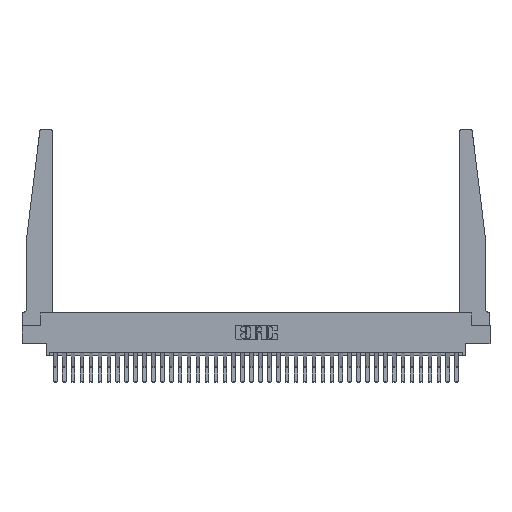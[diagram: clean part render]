
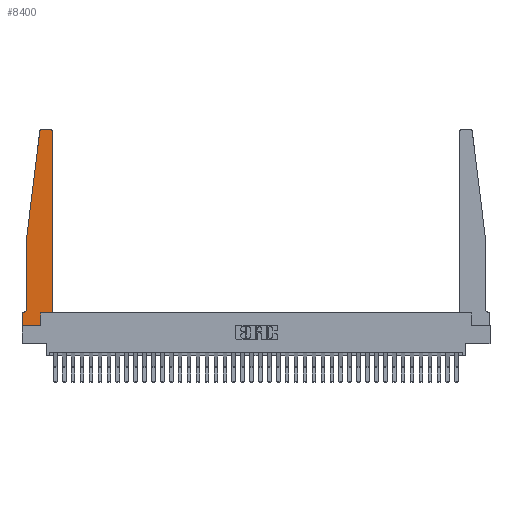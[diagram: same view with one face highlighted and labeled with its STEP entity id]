
A CAD part, top view. The second image highlights one B-rep face of the part: STEP entity #8400.
In plain terms, the highlighted planar face has unit normal (0, 0, 1).
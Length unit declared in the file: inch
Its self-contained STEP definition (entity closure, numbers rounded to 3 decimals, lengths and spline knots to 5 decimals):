
#57 = VERTEX_POINT ( 'NONE', #17377 ) ;
#651 = EDGE_CURVE ( 'NONE', #20871, #11792, #34197, .T. ) ;
#861 = ORIENTED_EDGE ( 'NONE', *, *, #651, .T. ) ;
#961 = VERTEX_POINT ( 'NONE', #33024 ) ;
#1134 = CARTESIAN_POINT ( 'NONE',  ( 0., 0., 0.37 ) ) ;
#1260 = DIRECTION ( 'NONE',  ( 0., 0., 1. ) ) ;
#1774 = CARTESIAN_POINT ( 'NONE',  ( 0.395, 2.72, 0.37 ) ) ;
#1888 = EDGE_CURVE ( 'NONE', #19231, #20515, #34127, .T. ) ;
#3084 = CARTESIAN_POINT ( 'NONE',  ( 0.2605, 0.18, 0.37 ) ) ;
#3683 = EDGE_CURVE ( 'NONE', #9748, #57, #34903, .T. ) ;
#3689 = CIRCLE ( 'NONE', #17245, 0.03 ) ;
#4533 = ORIENTED_EDGE ( 'NONE', *, *, #27854, .T. ) ;
#5013 = CARTESIAN_POINT ( 'NONE',  ( 0., 0., 0.37 ) ) ;
#5438 = ORIENTED_EDGE ( 'NONE', *, *, #30836, .T. ) ;
#5559 = DIRECTION ( 'NONE',  ( -1., 0., 0. ) ) ;
#6170 = VECTOR ( 'NONE', #18446, 39.37008 ) ;
#6265 = VECTOR ( 'NONE', #27032, 39.37008 ) ;
#6269 = VECTOR ( 'NONE', #11471, 39.37008 ) ;
#6580 = ORIENTED_EDGE ( 'NONE', *, *, #14342, .T. ) ;
#7221 = ORIENTED_EDGE ( 'NONE', *, *, #1888, .T. ) ;
#7347 = DIRECTION ( 'NONE',  ( 0., -1., 0. ) ) ;
#7409 = ORIENTED_EDGE ( 'NONE', *, *, #16816, .T. ) ;
#7435 = CARTESIAN_POINT ( 'NONE',  ( 0., 0.1875, 0.37 ) ) ;
#8255 = VERTEX_POINT ( 'NONE', #17357 ) ;
#8396 = CARTESIAN_POINT ( 'NONE',  ( 0.425, 0.18, 0.37 ) ) ;
#8400 = ADVANCED_FACE ( 'NONE', ( #10085 ), #17702, .T. ) ;
#8739 = VECTOR ( 'NONE', #32314, 39.37008 ) ;
#8923 = CARTESIAN_POINT ( 'NONE',  ( 0.065, 0.2375, 0.37 ) ) ;
#9300 = VECTOR ( 'NONE', #7347, 39.37008 ) ;
#9514 = EDGE_CURVE ( 'NONE', #20515, #18461, #20765, .T. ) ;
#9748 = VERTEX_POINT ( 'NONE', #33486 ) ;
#9895 = DIRECTION ( 'NONE',  ( -0.122, -0.992, 0. ) ) ;
#10085 = FACE_OUTER_BOUND ( 'NONE', #34365, .T. ) ;
#10113 = DIRECTION ( 'NONE',  ( 0., 1., 0. ) ) ;
#10686 = CARTESIAN_POINT ( 'NONE',  ( 0.065, 0.1875, 0.37 ) ) ;
#10743 = ORIENTED_EDGE ( 'NONE', *, *, #28792, .T. ) ;
#11127 = LINE ( 'NONE', #32678, #6269 ) ;
#11471 = DIRECTION ( 'NONE',  ( 0., 1., 0. ) ) ;
#11589 = VERTEX_POINT ( 'NONE', #3084 ) ;
#11792 = VERTEX_POINT ( 'NONE', #13082 ) ;
#12253 = LINE ( 'NONE', #22997, #18425 ) ;
#13082 = CARTESIAN_POINT ( 'NONE',  ( 0.395, 2.75, 0.37 ) ) ;
#13396 = CIRCLE ( 'NONE', #26358, 0.05 ) ;
#14103 = CARTESIAN_POINT ( 'NONE',  ( 0.065, 1.25, 0.37 ) ) ;
#14342 = EDGE_CURVE ( 'NONE', #18461, #9748, #13396, .T. ) ;
#15882 = LINE ( 'NONE', #26825, #8739 ) ;
#15974 = CARTESIAN_POINT ( 'NONE',  ( 0.425, 0.18, 0.37 ) ) ;
#16274 = CARTESIAN_POINT ( 'NONE',  ( 0.25, 2.75, 0.37 ) ) ;
#16376 = CARTESIAN_POINT ( 'NONE',  ( 0.425, 2.72, 0.37 ) ) ;
#16628 = VERTEX_POINT ( 'NONE', #1134 ) ;
#16816 = EDGE_CURVE ( 'NONE', #16628, #961, #26014, .T. ) ;
#17245 = AXIS2_PLACEMENT_3D ( 'NONE', #24487, #18039, #26136 ) ;
#17357 = CARTESIAN_POINT ( 'NONE',  ( 0.27653, 2.75, 0.37 ) ) ;
#17377 = CARTESIAN_POINT ( 'NONE',  ( 0., 0.1875, 0.37 ) ) ;
#17702 = PLANE ( 'NONE',  #33537 ) ;
#18039 = DIRECTION ( 'NONE',  ( 0., 0., 1. ) ) ;
#18086 = DIRECTION ( 'NONE',  ( -1., 0., 0. ) ) ;
#18353 = VECTOR ( 'NONE', #31691, 39.37008 ) ;
#18425 = VECTOR ( 'NONE', #10113, 39.37008 ) ;
#18446 = DIRECTION ( 'NONE',  ( 1., 0., 0. ) ) ;
#18461 = VERTEX_POINT ( 'NONE', #8923 ) ;
#18763 = EDGE_CURVE ( 'NONE', #11792, #8255, #24544, .T. ) ;
#18971 = ORIENTED_EDGE ( 'NONE', *, *, #3683, .T. ) ;
#19231 = VERTEX_POINT ( 'NONE', #28562 ) ;
#20515 = VERTEX_POINT ( 'NONE', #14103 ) ;
#20667 = CARTESIAN_POINT ( 'NONE',  ( 0.065, 1.25, 0.37 ) ) ;
#20765 = LINE ( 'NONE', #31537, #9300 ) ;
#20871 = VERTEX_POINT ( 'NONE', #16376 ) ;
#21637 = VECTOR ( 'NONE', #9895, 39.37008 ) ;
#21851 = EDGE_CURVE ( 'NONE', #961, #11589, #11127, .T. ) ;
#22798 = DIRECTION ( 'NONE',  ( 1., 0., 0. ) ) ;
#22997 = CARTESIAN_POINT ( 'NONE',  ( 0.425, 0.18, 0.37 ) ) ;
#23529 = CARTESIAN_POINT ( 'NONE',  ( 0.015, 0.2375, 0.37 ) ) ;
#23652 = VECTOR ( 'NONE', #5559, 39.37008 ) ;
#24487 = CARTESIAN_POINT ( 'NONE',  ( 0.27653, 2.72, 0.37 ) ) ;
#24544 = LINE ( 'NONE', #16274, #6265 ) ;
#25761 = AXIS2_PLACEMENT_3D ( 'NONE', #1774, #34647, #29304 ) ;
#26014 = LINE ( 'NONE', #5013, #6170 ) ;
#26136 = DIRECTION ( 'NONE',  ( 1., 0., 0. ) ) ;
#26290 = ORIENTED_EDGE ( 'NONE', *, *, #9514, .T. ) ;
#26358 = AXIS2_PLACEMENT_3D ( 'NONE', #23529, #31320, #18086 ) ;
#26825 = CARTESIAN_POINT ( 'NONE',  ( 0., 0., 0.37 ) ) ;
#27032 = DIRECTION ( 'NONE',  ( -1., 0., 0. ) ) ;
#27854 = EDGE_CURVE ( 'NONE', #57, #16628, #15882, .T. ) ;
#28562 = CARTESIAN_POINT ( 'NONE',  ( 0.24675, 2.72367, 0.37 ) ) ;
#28792 = EDGE_CURVE ( 'NONE', #11589, #34683, #32407, .T. ) ;
#29304 = DIRECTION ( 'NONE',  ( 1., 0., 0. ) ) ;
#30836 = EDGE_CURVE ( 'NONE', #8255, #19231, #3689, .T. ) ;
#31320 = DIRECTION ( 'NONE',  ( 0., 0., -1. ) ) ;
#31537 = CARTESIAN_POINT ( 'NONE',  ( 0.065, 1.25, 0.37 ) ) ;
#31691 = DIRECTION ( 'NONE',  ( 1., 0., 0. ) ) ;
#32005 = ORIENTED_EDGE ( 'NONE', *, *, #32008, .T. ) ;
#32008 = EDGE_CURVE ( 'NONE', #34683, #20871, #12253, .T. ) ;
#32314 = DIRECTION ( 'NONE',  ( 0., -1., 0. ) ) ;
#32407 = LINE ( 'NONE', #15974, #18353 ) ;
#32678 = CARTESIAN_POINT ( 'NONE',  ( 0.2605, 0.18, 0.37 ) ) ;
#33024 = CARTESIAN_POINT ( 'NONE',  ( 0.2605, 0., 0.37 ) ) ;
#33486 = CARTESIAN_POINT ( 'NONE',  ( 0.015, 0.1875, 0.37 ) ) ;
#33537 = AXIS2_PLACEMENT_3D ( 'NONE', #7435, #1260, #22798 ) ;
#34073 = ORIENTED_EDGE ( 'NONE', *, *, #18763, .T. ) ;
#34127 = LINE ( 'NONE', #20667, #21637 ) ;
#34197 = CIRCLE ( 'NONE', #25761, 0.03 ) ;
#34365 = EDGE_LOOP ( 'NONE', ( #34073, #5438, #7221, #26290, #6580, #18971, #4533, #7409, #34779, #10743, #32005, #861 ) ) ;
#34647 = DIRECTION ( 'NONE',  ( 0., 0., 1. ) ) ;
#34683 = VERTEX_POINT ( 'NONE', #8396 ) ;
#34779 = ORIENTED_EDGE ( 'NONE', *, *, #21851, .T. ) ;
#34903 = LINE ( 'NONE', #10686, #23652 ) ;
